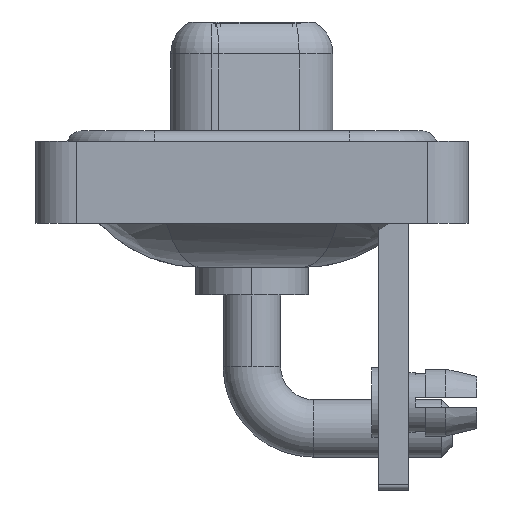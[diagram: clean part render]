
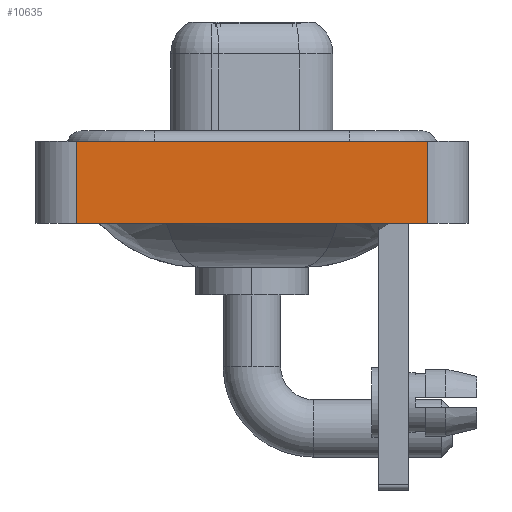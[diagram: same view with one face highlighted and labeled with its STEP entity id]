
A CAD part, left-side view. The second image highlights one B-rep face of the part: STEP entity #10635.
In plain terms, the highlighted planar face has unit normal (-1, 0, 0).
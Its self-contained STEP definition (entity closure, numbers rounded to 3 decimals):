
#1184 = LINE ( 'NONE', #14551, #17254 ) ;
#1570 = EDGE_CURVE ( 'NONE', #15582, #5935, #17938, .T. ) ;
#2426 = CARTESIAN_POINT ( 'NONE',  ( -7.35, 8.55, -3.6 ) ) ;
#2670 = EDGE_LOOP ( 'NONE', ( #11637, #8999, #16988, #4088 ) ) ;
#3802 = CARTESIAN_POINT ( 'NONE',  ( -7.35, 8.55, 0.4 ) ) ;
#3888 = CARTESIAN_POINT ( 'NONE',  ( -7.35, -8.55, -3.6 ) ) ;
#4088 = ORIENTED_EDGE ( 'NONE', *, *, #11437, .T. ) ;
#4514 = EDGE_CURVE ( 'NONE', #5935, #10929, #11521, .T. ) ;
#4853 = CARTESIAN_POINT ( 'NONE',  ( -7.35, 8.55, -3.6 ) ) ;
#5327 = VECTOR ( 'NONE', #15767, 1000. ) ;
#5748 = PLANE ( 'NONE',  #11995 ) ;
#5935 = VERTEX_POINT ( 'NONE', #3802 ) ;
#7260 = CARTESIAN_POINT ( 'NONE',  ( -7.35, -8.55, -3.6 ) ) ;
#7858 = DIRECTION ( 'NONE',  ( 0., 0., 1. ) ) ;
#8481 = DIRECTION ( 'NONE',  ( -1., 0., 0. ) ) ;
#8999 = ORIENTED_EDGE ( 'NONE', *, *, #4514, .F. ) ;
#9465 = VECTOR ( 'NONE', #11026, 1000. ) ;
#9598 = LINE ( 'NONE', #3888, #9465 ) ;
#9927 = CARTESIAN_POINT ( 'NONE',  ( -7.35, -8.55, -3.6 ) ) ;
#10635 = ADVANCED_FACE ( 'NONE', ( #17582 ), #5748, .T. ) ;
#10929 = VERTEX_POINT ( 'NONE', #17701 ) ;
#11026 = DIRECTION ( 'NONE',  ( 0., -1., 0. ) ) ;
#11437 = EDGE_CURVE ( 'NONE', #15582, #13175, #9598, .T. ) ;
#11521 = LINE ( 'NONE', #11705, #5327 ) ;
#11619 = DIRECTION ( 'NONE',  ( 0., 0., 1. ) ) ;
#11637 = ORIENTED_EDGE ( 'NONE', *, *, #15603, .T. ) ;
#11705 = CARTESIAN_POINT ( 'NONE',  ( -7.35, -8.55, 0.4 ) ) ;
#11995 = AXIS2_PLACEMENT_3D ( 'NONE', #9927, #8481, #11619 ) ;
#13175 = VERTEX_POINT ( 'NONE', #7260 ) ;
#14320 = VECTOR ( 'NONE', #7858, 1000. ) ;
#14366 = DIRECTION ( 'NONE',  ( 0., 0., 1. ) ) ;
#14551 = CARTESIAN_POINT ( 'NONE',  ( -7.35, -8.55, -3.6 ) ) ;
#15582 = VERTEX_POINT ( 'NONE', #2426 ) ;
#15603 = EDGE_CURVE ( 'NONE', #13175, #10929, #1184, .T. ) ;
#15767 = DIRECTION ( 'NONE',  ( 0., -1., 0. ) ) ;
#16988 = ORIENTED_EDGE ( 'NONE', *, *, #1570, .F. ) ;
#17254 = VECTOR ( 'NONE', #14366, 1000. ) ;
#17582 = FACE_OUTER_BOUND ( 'NONE', #2670, .T. ) ;
#17701 = CARTESIAN_POINT ( 'NONE',  ( -7.35, -8.55, 0.4 ) ) ;
#17938 = LINE ( 'NONE', #4853, #14320 ) ;
